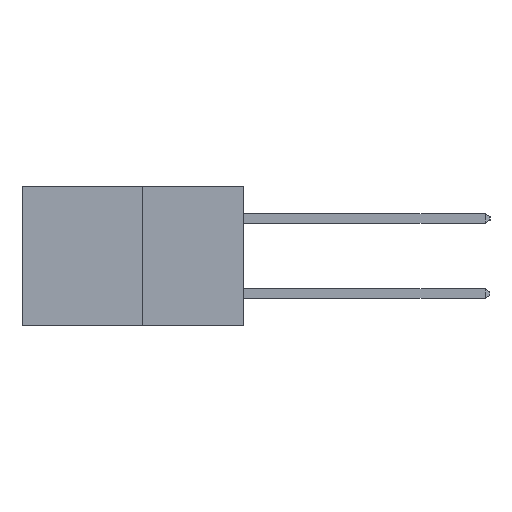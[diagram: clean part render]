
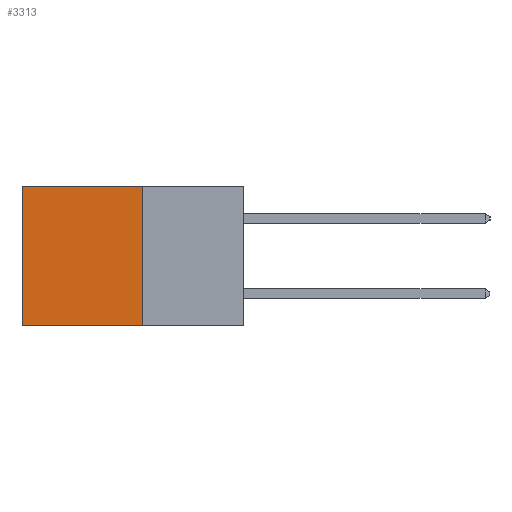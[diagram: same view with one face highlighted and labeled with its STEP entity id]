
A CAD part, left-side view. The second image highlights one B-rep face of the part: STEP entity #3313.
In plain terms, the highlighted planar face has unit normal (-1, 0, 0).
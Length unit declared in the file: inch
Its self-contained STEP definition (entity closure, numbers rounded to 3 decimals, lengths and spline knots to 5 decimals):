
#448 = EDGE_CURVE ( 'NONE', #8242, #5251, #6087, .T. ) ;
#478 = EDGE_LOOP ( 'NONE', ( #12696, #3885, #1797, #6692 ) ) ;
#596 = DIRECTION ( 'NONE',  ( 0., 1., 0. ) ) ;
#964 = DIRECTION ( 'NONE',  ( 0., 0., -1. ) ) ;
#1408 = CARTESIAN_POINT ( 'NONE',  ( 0.277, 0.59, 0. ) ) ;
#1572 = VERTEX_POINT ( 'NONE', #1408 ) ;
#1640 = VECTOR ( 'NONE', #596, 39.37008 ) ;
#1797 = ORIENTED_EDGE ( 'NONE', *, *, #448, .F. ) ;
#1945 = EDGE_CURVE ( 'NONE', #8242, #1572, #10215, .T. ) ;
#1956 = DIRECTION ( 'NONE',  ( 0., 0., -1. ) ) ;
#3183 = VECTOR ( 'NONE', #1956, 39.37008 ) ;
#3313 = ADVANCED_FACE ( 'NONE', ( #12627 ), #8760, .F. ) ;
#3885 = ORIENTED_EDGE ( 'NONE', *, *, #5450, .F. ) ;
#5251 = VERTEX_POINT ( 'NONE', #6141 ) ;
#5450 = EDGE_CURVE ( 'NONE', #5251, #9054, #12049, .T. ) ;
#5702 = EDGE_CURVE ( 'NONE', #1572, #9054, #6344, .T. ) ;
#6087 = LINE ( 'NONE', #10718, #3183 ) ;
#6141 = CARTESIAN_POINT ( 'NONE',  ( 0.277, 0.27, -0.37 ) ) ;
#6344 = LINE ( 'NONE', #6787, #11577 ) ;
#6685 = CARTESIAN_POINT ( 'NONE',  ( 0.277, 0.27, 0. ) ) ;
#6692 = ORIENTED_EDGE ( 'NONE', *, *, #1945, .T. ) ;
#6787 = CARTESIAN_POINT ( 'NONE',  ( 0.277, 0.59, -0.37 ) ) ;
#7844 = VECTOR ( 'NONE', #8740, 39.37008 ) ;
#8242 = VERTEX_POINT ( 'NONE', #9217 ) ;
#8720 = DIRECTION ( 'NONE',  ( 0., 0., -1. ) ) ;
#8726 = DIRECTION ( 'NONE',  ( 1., 0., 0. ) ) ;
#8740 = DIRECTION ( 'NONE',  ( 0., 1., 0. ) ) ;
#8760 = PLANE ( 'NONE',  #12680 ) ;
#9035 = CARTESIAN_POINT ( 'NONE',  ( 0.277, 0.27, -0.37 ) ) ;
#9054 = VERTEX_POINT ( 'NONE', #10375 ) ;
#9217 = CARTESIAN_POINT ( 'NONE',  ( 0.277, 0.27, 0. ) ) ;
#10215 = LINE ( 'NONE', #6685, #7844 ) ;
#10375 = CARTESIAN_POINT ( 'NONE',  ( 0.277, 0.59, -0.37 ) ) ;
#10387 = CARTESIAN_POINT ( 'NONE',  ( 0.277, 0.27, -0.37 ) ) ;
#10718 = CARTESIAN_POINT ( 'NONE',  ( 0.277, 0.27, -0.37 ) ) ;
#11577 = VECTOR ( 'NONE', #964, 39.37008 ) ;
#12049 = LINE ( 'NONE', #10387, #1640 ) ;
#12627 = FACE_OUTER_BOUND ( 'NONE', #478, .T. ) ;
#12680 = AXIS2_PLACEMENT_3D ( 'NONE', #9035, #8726, #8720 ) ;
#12696 = ORIENTED_EDGE ( 'NONE', *, *, #5702, .T. ) ;
